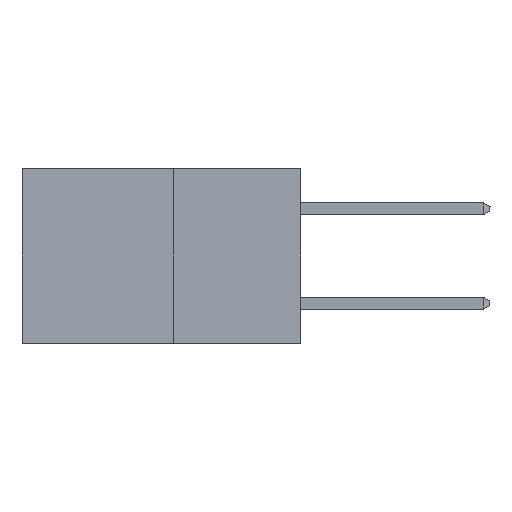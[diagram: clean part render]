
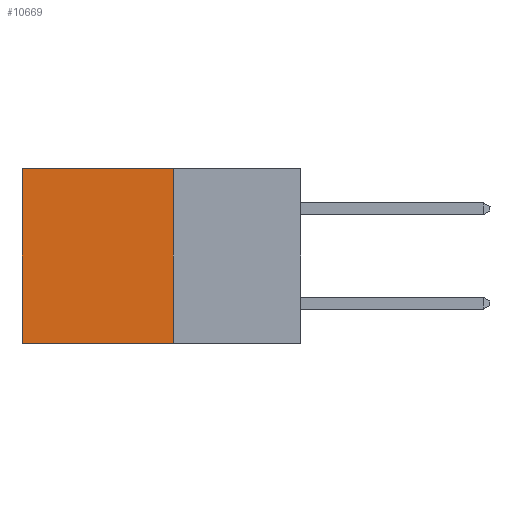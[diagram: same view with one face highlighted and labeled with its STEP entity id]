
A CAD part, left-side view. The second image highlights one B-rep face of the part: STEP entity #10669.
In plain terms, the highlighted planar face has unit normal (-1, 0, 0).
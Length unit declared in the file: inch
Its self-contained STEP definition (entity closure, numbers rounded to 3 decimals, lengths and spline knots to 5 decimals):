
#27 = EDGE_CURVE ( 'NONE', #13518, #5744, #9533, .T. ) ;
#376 = VECTOR ( 'NONE', #6015, 39.37008 ) ;
#1156 = DIRECTION ( 'NONE',  ( 0., 1., 0. ) ) ;
#1186 = ORIENTED_EDGE ( 'NONE', *, *, #5741, .T. ) ;
#1212 = ORIENTED_EDGE ( 'NONE', *, *, #8003, .F. ) ;
#1379 = ORIENTED_EDGE ( 'NONE', *, *, #10164, .F. ) ;
#1416 = ORIENTED_EDGE ( 'NONE', *, *, #27, .T. ) ;
#1690 = VECTOR ( 'NONE', #1156, 39.37008 ) ;
#2032 = VERTEX_POINT ( 'NONE', #13325 ) ;
#2969 = CARTESIAN_POINT ( 'NONE',  ( 0.277, 0.27, -0.37 ) ) ;
#2994 = CARTESIAN_POINT ( 'NONE',  ( 0.277, 0.59, 0. ) ) ;
#3736 = EDGE_LOOP ( 'NONE', ( #1186, #1212, #1379, #1416 ) ) ;
#3903 = PLANE ( 'NONE',  #10123 ) ;
#3955 = VECTOR ( 'NONE', #5635, 39.37008 ) ;
#4351 = FACE_OUTER_BOUND ( 'NONE', #3736, .T. ) ;
#4496 = CARTESIAN_POINT ( 'NONE',  ( 0.277, 0.27, -0.37 ) ) ;
#4820 = CARTESIAN_POINT ( 'NONE',  ( 0.277, 0.59, -0.37 ) ) ;
#4913 = DIRECTION ( 'NONE',  ( 1., 0., 0. ) ) ;
#5432 = CARTESIAN_POINT ( 'NONE',  ( 0.277, 0.27, -0.37 ) ) ;
#5635 = DIRECTION ( 'NONE',  ( 0., 1., 0. ) ) ;
#5741 = EDGE_CURVE ( 'NONE', #5744, #2032, #11643, .T. ) ;
#5744 = VERTEX_POINT ( 'NONE', #2994 ) ;
#6015 = DIRECTION ( 'NONE',  ( 0., 0., -1. ) ) ;
#6599 = CARTESIAN_POINT ( 'NONE',  ( 0.277, 0.27, 0. ) ) ;
#6785 = DIRECTION ( 'NONE',  ( 0., 0., -1. ) ) ;
#8003 = EDGE_CURVE ( 'NONE', #8031, #2032, #9681, .T. ) ;
#8031 = VERTEX_POINT ( 'NONE', #4496 ) ;
#8113 = CARTESIAN_POINT ( 'NONE',  ( 0.277, 0.27, -0.37 ) ) ;
#8372 = CARTESIAN_POINT ( 'NONE',  ( 0.277, 0.27, 0. ) ) ;
#9533 = LINE ( 'NONE', #8372, #1690 ) ;
#9681 = LINE ( 'NONE', #5432, #3955 ) ;
#10123 = AXIS2_PLACEMENT_3D ( 'NONE', #8113, #4913, #12468 ) ;
#10164 = EDGE_CURVE ( 'NONE', #13518, #8031, #11791, .T. ) ;
#10669 = ADVANCED_FACE ( 'NONE', ( #4351 ), #3903, .F. ) ;
#11306 = VECTOR ( 'NONE', #6785, 39.37008 ) ;
#11643 = LINE ( 'NONE', #4820, #11306 ) ;
#11791 = LINE ( 'NONE', #2969, #376 ) ;
#12468 = DIRECTION ( 'NONE',  ( 0., 0., -1. ) ) ;
#13325 = CARTESIAN_POINT ( 'NONE',  ( 0.277, 0.59, -0.37 ) ) ;
#13518 = VERTEX_POINT ( 'NONE', #6599 ) ;
